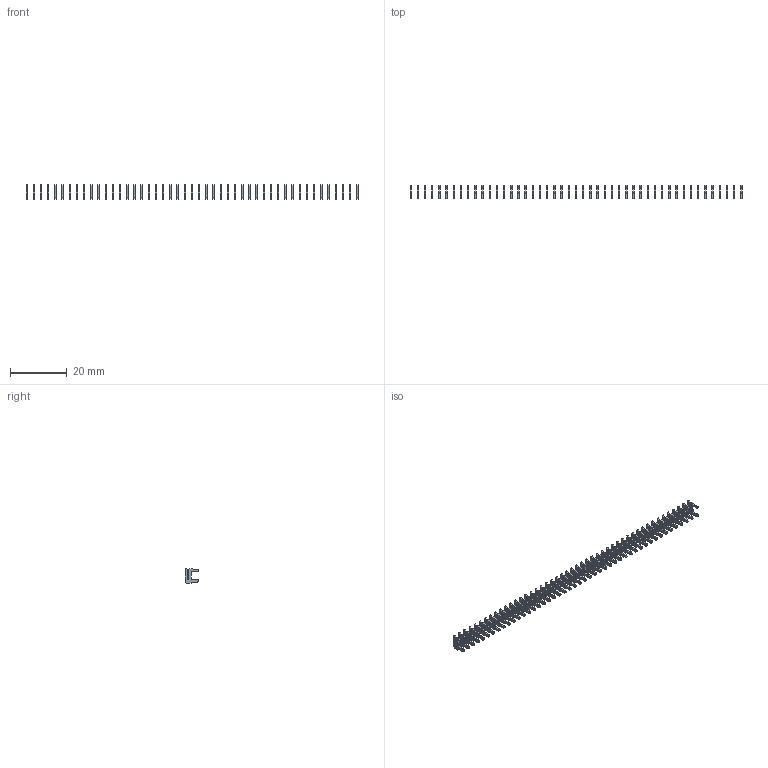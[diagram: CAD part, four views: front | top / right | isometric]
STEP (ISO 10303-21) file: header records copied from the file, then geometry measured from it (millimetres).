
FILE_DESCRIPTION (( 'STEP AP203' ), '1' );
FILE_NAME ('105-047-208-100.STEP', '2020-04-08T00:18:07', ( '' ), ( '' ), 'SwSTEP 2.0', 'SolidWorks 2016', '' );
FILE_SCHEMA (( 'CONFIG_CONTROL_DESIGN' ));
Length unit declared in the file: inch
Products named in the file (2): 100-290-001_100-290-208; 105-047-208-100
Assembly tree (47 placements, depth 2):
  105-047-208-100
    100-290-001_100-290-208  x47
Bounding box: 117.35 x 4.83 x 5.17 mm (x, y, z)
Volume: 323.4 mm3; surface area: 1997.3 mm2
Topology: 47 solids, 47 shells, 1175 faces, 3243 edges, 2162 vertices
Faces by surface type: plane 1034, cylinder 141
Entity records: 2461 total; most frequent: DIRECTION 225, CARTESIAN_POINT 190, ORIENTED_EDGE 138, CALENDAR_DATE 104, COORDINATED_UNIVERSAL_TIME_OFFSET 104, DATE_AND_TIME 104, LOCAL_TIME 104, AXIS2_PLACEMENT_3D 81
